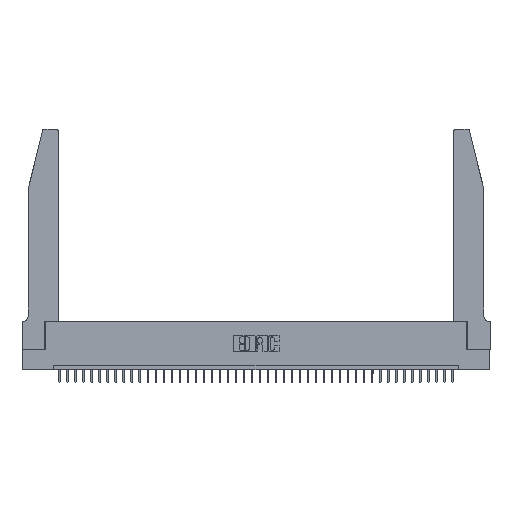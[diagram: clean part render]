
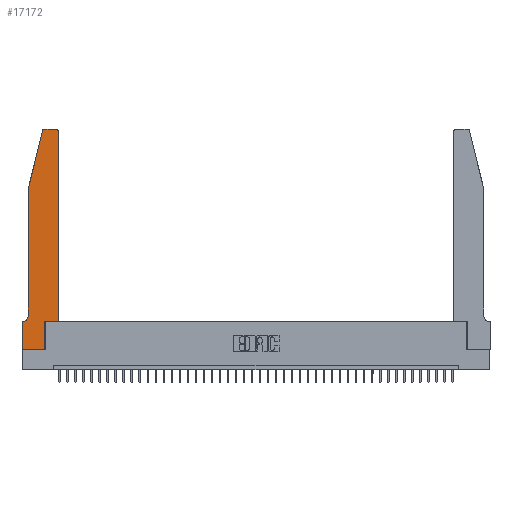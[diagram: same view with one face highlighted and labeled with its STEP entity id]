
A CAD part, top view. The second image highlights one B-rep face of the part: STEP entity #17172.
In plain terms, the highlighted planar face has unit normal (0, 0, 1).
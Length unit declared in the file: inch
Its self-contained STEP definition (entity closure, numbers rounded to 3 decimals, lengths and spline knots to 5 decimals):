
#153 = EDGE_CURVE ( 'NONE', #32008, #9035, #15314, .T. ) ;
#570 = ORIENTED_EDGE ( 'NONE', *, *, #29087, .T. ) ;
#788 = VERTEX_POINT ( 'NONE', #9444 ) ;
#828 = CARTESIAN_POINT ( 'NONE',  ( 0.0755, 2., 0.37 ) ) ;
#1133 = DIRECTION ( 'NONE',  ( 0., -1., 0. ) ) ;
#1214 = ORIENTED_EDGE ( 'NONE', *, *, #10551, .T. ) ;
#1541 = LINE ( 'NONE', #29314, #31524 ) ;
#3206 = CARTESIAN_POINT ( 'NONE',  ( 0.4505, 0.35, 0.37 ) ) ;
#4076 = DIRECTION ( 'NONE',  ( 0., -1., 0. ) ) ;
#4766 = LINE ( 'NONE', #36567, #40250 ) ;
#5429 = AXIS2_PLACEMENT_3D ( 'NONE', #31262, #13038, #22671 ) ;
#5472 = EDGE_CURVE ( 'NONE', #18729, #788, #37365, .T. ) ;
#6628 = CARTESIAN_POINT ( 'NONE',  ( 0., 0., 0.37 ) ) ;
#6644 = CARTESIAN_POINT ( 'NONE',  ( 0.4205, 2.75, 0.37 ) ) ;
#6826 = DIRECTION ( 'NONE',  ( 1., 0., 0. ) ) ;
#7466 = EDGE_CURVE ( 'NONE', #17807, #25535, #20119, .T. ) ;
#7816 = DIRECTION ( 'NONE',  ( 0., 1., 0. ) ) ;
#8397 = CARTESIAN_POINT ( 'NONE',  ( 0.2865, 0., 0.37 ) ) ;
#8556 = EDGE_CURVE ( 'NONE', #21035, #28710, #39538, .T. ) ;
#8743 = AXIS2_PLACEMENT_3D ( 'NONE', #30567, #18180, #15094 ) ;
#9035 = VERTEX_POINT ( 'NONE', #15624 ) ;
#9444 = CARTESIAN_POINT ( 'NONE',  ( 0.0755, 2., 0.37 ) ) ;
#9938 = DIRECTION ( 'NONE',  ( 1., 0., 0. ) ) ;
#10087 = CARTESIAN_POINT ( 'NONE',  ( 0.2865, 0.35, 0.37 ) ) ;
#10345 = AXIS2_PLACEMENT_3D ( 'NONE', #22801, #25446, #16628 ) ;
#10533 = DIRECTION ( 'NONE',  ( 0., 0., 1. ) ) ;
#10551 = EDGE_CURVE ( 'NONE', #40936, #17807, #26808, .T. ) ;
#11131 = ORIENTED_EDGE ( 'NONE', *, *, #16464, .T. ) ;
#12283 = VECTOR ( 'NONE', #30969, 39.37008 ) ;
#12312 = VERTEX_POINT ( 'NONE', #8397 ) ;
#13038 = DIRECTION ( 'NONE',  ( 0., 0., 1. ) ) ;
#13636 = DIRECTION ( 'NONE',  ( 0., 1., 0. ) ) ;
#14225 = ORIENTED_EDGE ( 'NONE', *, *, #153, .T. ) ;
#14516 = PLANE ( 'NONE',  #8743 ) ;
#15094 = DIRECTION ( 'NONE',  ( 1., 0., 0. ) ) ;
#15166 = LINE ( 'NONE', #828, #27121 ) ;
#15314 = LINE ( 'NONE', #34459, #12283 ) ;
#15623 = CARTESIAN_POINT ( 'NONE',  ( 0., 0., 0.37 ) ) ;
#15624 = CARTESIAN_POINT ( 'NONE',  ( 0., 0.35, 0.37 ) ) ;
#15837 = LINE ( 'NONE', #17314, #34356 ) ;
#16376 = CARTESIAN_POINT ( 'NONE',  ( 0.0755, 0.42, 0.37 ) ) ;
#16464 = EDGE_CURVE ( 'NONE', #788, #30420, #15166, .T. ) ;
#16479 = ORIENTED_EDGE ( 'NONE', *, *, #7466, .T. ) ;
#16628 = DIRECTION ( 'NONE',  ( -1., 0., 0. ) ) ;
#16849 = CARTESIAN_POINT ( 'NONE',  ( 0.284, 2.72, 0.37 ) ) ;
#17172 = ADVANCED_FACE ( 'NONE', ( #26061 ), #14516, .T. ) ;
#17314 = CARTESIAN_POINT ( 'NONE',  ( 0.2865, 0.35, 0.37 ) ) ;
#17441 = DIRECTION ( 'NONE',  ( -0.239, -0.971, 0. ) ) ;
#17807 = VERTEX_POINT ( 'NONE', #6644 ) ;
#18180 = DIRECTION ( 'NONE',  ( 0., 0., 1. ) ) ;
#18318 = EDGE_CURVE ( 'NONE', #21664, #12312, #28514, .T. ) ;
#18729 = VERTEX_POINT ( 'NONE', #31187 ) ;
#19435 = CARTESIAN_POINT ( 'NONE',  ( 0.4505, 0.35, 0.37 ) ) ;
#19897 = EDGE_LOOP ( 'NONE', ( #16479, #37960, #35804, #11131, #32846, #14225, #570, #38381, #38968, #34154, #35258, #1214 ) ) ;
#20119 = LINE ( 'NONE', #25317, #35128 ) ;
#21035 = VERTEX_POINT ( 'NONE', #10087 ) ;
#21664 = VERTEX_POINT ( 'NONE', #6628 ) ;
#22671 = DIRECTION ( 'NONE',  ( 1., 0., 0. ) ) ;
#22801 = CARTESIAN_POINT ( 'NONE',  ( 0.0055, 0.42, 0.37 ) ) ;
#23114 = CARTESIAN_POINT ( 'NONE',  ( 0.4505, 2.72, 0.37 ) ) ;
#23505 = VECTOR ( 'NONE', #9938, 39.37008 ) ;
#24837 = VECTOR ( 'NONE', #17441, 39.37008 ) ;
#25253 = DIRECTION ( 'NONE',  ( 1., 0., 0. ) ) ;
#25317 = CARTESIAN_POINT ( 'NONE',  ( 0.2605, 2.75, 0.37 ) ) ;
#25446 = DIRECTION ( 'NONE',  ( 0., 0., -1. ) ) ;
#25464 = DIRECTION ( 'NONE',  ( -1., 0., 0. ) ) ;
#25535 = VERTEX_POINT ( 'NONE', #27265 ) ;
#25550 = CIRCLE ( 'NONE', #10345, 0.07 ) ;
#26061 = FACE_OUTER_BOUND ( 'NONE', #19897, .T. ) ;
#26158 = AXIS2_PLACEMENT_3D ( 'NONE', #16849, #10533, #6826 ) ;
#26683 = EDGE_CURVE ( 'NONE', #28710, #40936, #4766, .T. ) ;
#26808 = CIRCLE ( 'NONE', #5429, 0.03 ) ;
#26925 = CARTESIAN_POINT ( 'NONE',  ( 0.0755, 2., 0.37 ) ) ;
#27121 = VECTOR ( 'NONE', #4076, 39.37008 ) ;
#27265 = CARTESIAN_POINT ( 'NONE',  ( 0.284, 2.75, 0.37 ) ) ;
#28082 = EDGE_CURVE ( 'NONE', #25535, #18729, #39075, .T. ) ;
#28514 = LINE ( 'NONE', #15623, #38487 ) ;
#28602 = EDGE_CURVE ( 'NONE', #30420, #32008, #25550, .T. ) ;
#28710 = VERTEX_POINT ( 'NONE', #3206 ) ;
#29087 = EDGE_CURVE ( 'NONE', #9035, #21664, #1541, .T. ) ;
#29314 = CARTESIAN_POINT ( 'NONE',  ( 0., 0., 0.37 ) ) ;
#30420 = VERTEX_POINT ( 'NONE', #16376 ) ;
#30567 = CARTESIAN_POINT ( 'NONE',  ( 0., 0.35, 0.37 ) ) ;
#30969 = DIRECTION ( 'NONE',  ( -1., 0., 0. ) ) ;
#31187 = CARTESIAN_POINT ( 'NONE',  ( 0.25487, 2.72718, 0.37 ) ) ;
#31262 = CARTESIAN_POINT ( 'NONE',  ( 0.4205, 2.72, 0.37 ) ) ;
#31524 = VECTOR ( 'NONE', #1133, 39.37008 ) ;
#32008 = VERTEX_POINT ( 'NONE', #33886 ) ;
#32846 = ORIENTED_EDGE ( 'NONE', *, *, #28602, .T. ) ;
#33886 = CARTESIAN_POINT ( 'NONE',  ( 0.0055, 0.35, 0.37 ) ) ;
#34154 = ORIENTED_EDGE ( 'NONE', *, *, #8556, .T. ) ;
#34356 = VECTOR ( 'NONE', #7816, 39.37008 ) ;
#34459 = CARTESIAN_POINT ( 'NONE',  ( 0.0755, 0.35, 0.37 ) ) ;
#35128 = VECTOR ( 'NONE', #25464, 39.37008 ) ;
#35258 = ORIENTED_EDGE ( 'NONE', *, *, #26683, .T. ) ;
#35804 = ORIENTED_EDGE ( 'NONE', *, *, #5472, .T. ) ;
#36567 = CARTESIAN_POINT ( 'NONE',  ( 0.4505, 0.35, 0.37 ) ) ;
#37090 = EDGE_CURVE ( 'NONE', #12312, #21035, #15837, .T. ) ;
#37365 = LINE ( 'NONE', #26925, #24837 ) ;
#37960 = ORIENTED_EDGE ( 'NONE', *, *, #28082, .T. ) ;
#38381 = ORIENTED_EDGE ( 'NONE', *, *, #18318, .T. ) ;
#38487 = VECTOR ( 'NONE', #25253, 39.37008 ) ;
#38968 = ORIENTED_EDGE ( 'NONE', *, *, #37090, .T. ) ;
#39075 = CIRCLE ( 'NONE', #26158, 0.03 ) ;
#39538 = LINE ( 'NONE', #19435, #23505 ) ;
#40250 = VECTOR ( 'NONE', #13636, 39.37008 ) ;
#40936 = VERTEX_POINT ( 'NONE', #23114 ) ;
